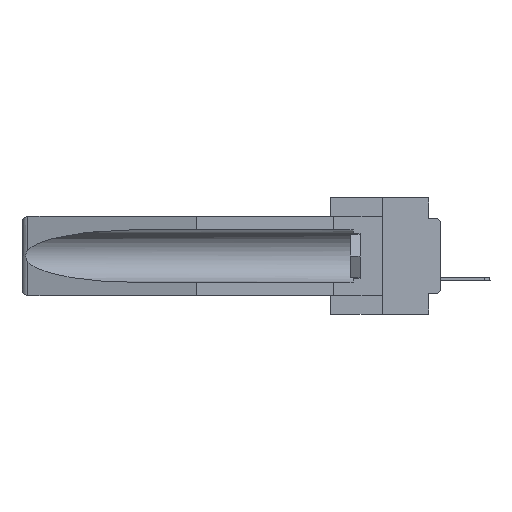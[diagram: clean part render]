
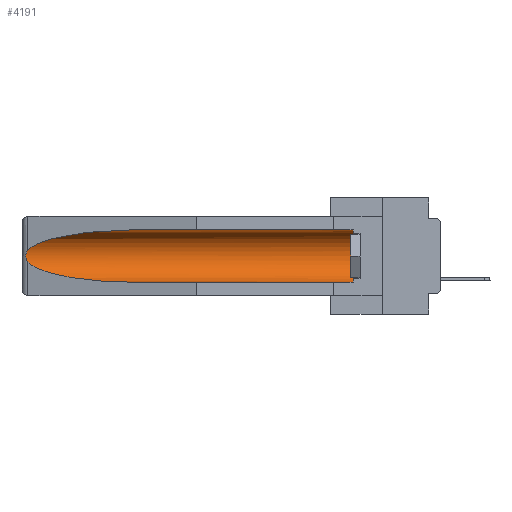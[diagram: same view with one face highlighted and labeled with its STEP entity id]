
A CAD part, left-side view. The second image highlights one B-rep face of the part: STEP entity #4191.
In plain terms, the highlighted cylindrical face has radius 2.857 mm (diameter 5.715 mm), a partial arc.
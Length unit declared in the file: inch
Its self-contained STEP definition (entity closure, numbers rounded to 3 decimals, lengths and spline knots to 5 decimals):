
#304 = EDGE_CURVE ( 'NONE', #6528, #14476, #13437, .T. ) ;
#364 = CARTESIAN_POINT ( 'NONE',  ( 0.26537, 1.52718, -0.14972 ) ) ;
#723 = CARTESIAN_POINT ( 'NONE',  ( 0.155, 1.07973, -0.059 ) ) ;
#934 = FACE_OUTER_BOUND ( 'NONE', #5259, .T. ) ;
#1654 = VERTEX_POINT ( 'NONE', #28830 ) ;
#1934 = AXIS2_PLACEMENT_3D ( 'NONE', #33872, #25604, #9256 ) ;
#2189 = CARTESIAN_POINT ( 'NONE',  ( 0.26537, 1.52718, -0.19328 ) ) ;
#4030 = CARTESIAN_POINT ( 'NONE',  ( 0.26537, 1.52718, -0.19328 ) ) ;
#4191 = ADVANCED_FACE ( 'NONE', ( #934 ), #14422, .F. ) ;
#5258 = ORIENTED_EDGE ( 'NONE', *, *, #30575, .F. ) ;
#5259 = EDGE_LOOP ( 'NONE', ( #13087, #17133, #25161, #5258, #21989, #18502 ) ) ;
#6166 = DIRECTION ( 'NONE',  ( 0., 1., 0. ) ) ;
#6495 = CARTESIAN_POINT ( 'NONE',  ( 0.26654, 1.53092, -0.15636 ) ) ;
#6528 = VERTEX_POINT ( 'NONE', #16189 ) ;
#7386 = LINE ( 'NONE', #18347, #11697 ) ;
#9137 = VERTEX_POINT ( 'NONE', #364 ) ;
#9256 = DIRECTION ( 'NONE',  ( 0., 0., 1. ) ) ;
#10519 = CARTESIAN_POINT ( 'NONE',  ( 0.155, 0.126, -0.059 ) ) ;
#10520 = EDGE_CURVE ( 'NONE', #1654, #33908, #31205, .T. ) ;
#10859 = EDGE_CURVE ( 'NONE', #34798, #9137, #11278, .T. ) ;
#11278 =( BOUNDED_CURVE ( )  B_SPLINE_CURVE ( 3, ( #723, #17621, #34312, #25514 ),
 .UNSPECIFIED., .F., .T. ) 
 B_SPLINE_CURVE_WITH_KNOTS ( ( 4, 4 ),
 ( 4.71239, 6.08839 ),
 .UNSPECIFIED. ) 
 CURVE ( )  GEOMETRIC_REPRESENTATION_ITEM ( )  RATIONAL_B_SPLINE_CURVE ( ( 1., 0.848, 0.848, 1. ) ) 
 REPRESENTATION_ITEM ( '' )  );
#11697 = VECTOR ( 'NONE', #34514, 39.37008 ) ;
#13087 = ORIENTED_EDGE ( 'NONE', *, *, #10859, .T. ) ;
#13161 = CARTESIAN_POINT ( 'NONE',  ( 0.155, 1.07973, -0.284 ) ) ;
#13437 = CIRCLE ( 'NONE', #1934, 0.1125 ) ;
#14422 = CYLINDRICAL_SURFACE ( 'NONE', #28583, 0.1125 ) ;
#14476 = VERTEX_POINT ( 'NONE', #10519 ) ;
#15495 = CARTESIAN_POINT ( 'NONE',  ( 0.21114, 1.30732, -0.284 ) ) ;
#16189 = CARTESIAN_POINT ( 'NONE',  ( 0.155, 0.126, -0.284 ) ) ;
#17133 = ORIENTED_EDGE ( 'NONE', *, *, #22778, .T. ) ;
#17621 = CARTESIAN_POINT ( 'NONE',  ( 0.21114, 1.30732, -0.059 ) ) ;
#18212 = CARTESIAN_POINT ( 'NONE',  ( 0.2675, 1.53308, -0.16763 ) ) ;
#18347 = CARTESIAN_POINT ( 'NONE',  ( 0.155, -0.30754, -0.059 ) ) ;
#18502 = ORIENTED_EDGE ( 'NONE', *, *, #21892, .T. ) ;
#20399 = CARTESIAN_POINT ( 'NONE',  ( 0.155, -0.30754, -0.284 ) ) ;
#20543 = CARTESIAN_POINT ( 'NONE',  ( 0.26655, 1.53094, -0.18657 ) ) ;
#21892 = EDGE_CURVE ( 'NONE', #14476, #34798, #7386, .T. ) ;
#21989 = ORIENTED_EDGE ( 'NONE', *, *, #304, .T. ) ;
#22778 = EDGE_CURVE ( 'NONE', #9137, #1654, #23089, .T. ) ;
#23089 = B_SPLINE_CURVE_WITH_KNOTS ( 'NONE', 3,
 ( #31124, #24342, #6495, #35301, #18212, #23411, #34382, #20543, #34557, #4030 ),
 .UNSPECIFIED., .F., .F.,
 ( 4, 2, 2, 2, 4 ),
 ( 0., 0.00029, 0.00058, 0.00087, 0.00117 ),
 .UNSPECIFIED. ) ;
#23411 = CARTESIAN_POINT ( 'NONE',  ( 0.2675, 1.53308, -0.17534 ) ) ;
#24308 = CARTESIAN_POINT ( 'NONE',  ( 0.155, 1.07973, -0.284 ) ) ;
#24342 = CARTESIAN_POINT ( 'NONE',  ( 0.26597, 1.52961, -0.15275 ) ) ;
#25161 = ORIENTED_EDGE ( 'NONE', *, *, #10520, .T. ) ;
#25514 = CARTESIAN_POINT ( 'NONE',  ( 0.26537, 1.52718, -0.14972 ) ) ;
#25604 = DIRECTION ( 'NONE',  ( 0., -1., 0. ) ) ;
#28069 = CARTESIAN_POINT ( 'NONE',  ( 0.155, -0.30754, -0.1715 ) ) ;
#28423 = DIRECTION ( 'NONE',  ( 0., 0., 1. ) ) ;
#28583 = AXIS2_PLACEMENT_3D ( 'NONE', #28069, #6166, #28423 ) ;
#28830 = CARTESIAN_POINT ( 'NONE',  ( 0.26537, 1.52718, -0.19328 ) ) ;
#28840 = DIRECTION ( 'NONE',  ( 0., 1., 0. ) ) ;
#30575 = EDGE_CURVE ( 'NONE', #6528, #33908, #31380, .T. ) ;
#31124 = CARTESIAN_POINT ( 'NONE',  ( 0.26537, 1.52718, -0.14972 ) ) ;
#31205 =( BOUNDED_CURVE ( )  B_SPLINE_CURVE ( 3, ( #2189, #32023, #15495, #13161 ),
 .UNSPECIFIED., .F., .F. ) 
 B_SPLINE_CURVE_WITH_KNOTS ( ( 4, 4 ),
 ( 0.1948, 1.5708 ),
 .UNSPECIFIED. ) 
 CURVE ( )  GEOMETRIC_REPRESENTATION_ITEM ( )  RATIONAL_B_SPLINE_CURVE ( ( 1., 0.848, 0.848, 1. ) ) 
 REPRESENTATION_ITEM ( '' )  );
#31380 = LINE ( 'NONE', #20399, #34732 ) ;
#32023 = CARTESIAN_POINT ( 'NONE',  ( 0.25451, 1.48313, -0.24835 ) ) ;
#33872 = CARTESIAN_POINT ( 'NONE',  ( 0.155, 0.126, -0.1715 ) ) ;
#33908 = VERTEX_POINT ( 'NONE', #24308 ) ;
#34312 = CARTESIAN_POINT ( 'NONE',  ( 0.25451, 1.48313, -0.09465 ) ) ;
#34382 = CARTESIAN_POINT ( 'NONE',  ( 0.2673, 1.53269, -0.17917 ) ) ;
#34514 = DIRECTION ( 'NONE',  ( 0., 1., 0. ) ) ;
#34557 = CARTESIAN_POINT ( 'NONE',  ( 0.26597, 1.5296, -0.19026 ) ) ;
#34732 = VECTOR ( 'NONE', #28840, 39.37008 ) ;
#34798 = VERTEX_POINT ( 'NONE', #35316 ) ;
#35301 = CARTESIAN_POINT ( 'NONE',  ( 0.2673, 1.5327, -0.16383 ) ) ;
#35316 = CARTESIAN_POINT ( 'NONE',  ( 0.155, 1.07973, -0.059 ) ) ;
